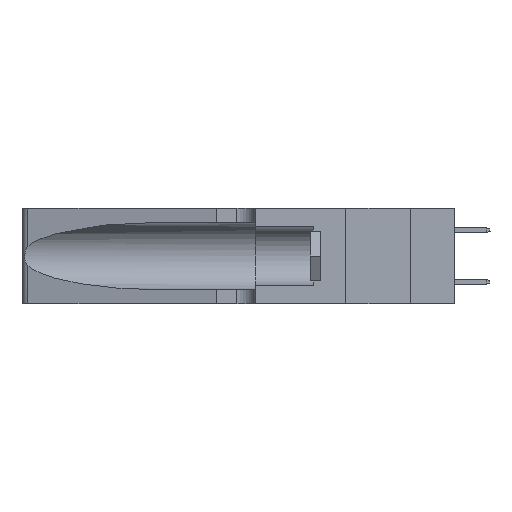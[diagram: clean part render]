
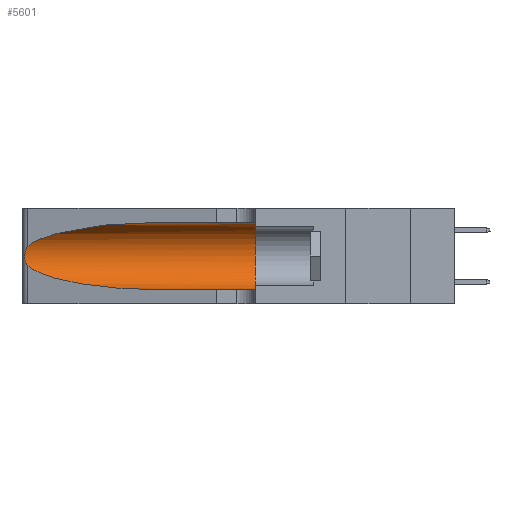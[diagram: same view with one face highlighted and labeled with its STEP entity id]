
A CAD part, left-side view. The second image highlights one B-rep face of the part: STEP entity #5601.
In plain terms, the highlighted cylindrical face has radius 3.308 mm (diameter 6.617 mm), a partial arc.
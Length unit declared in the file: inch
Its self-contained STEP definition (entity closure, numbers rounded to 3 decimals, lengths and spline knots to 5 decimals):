
#355 = DIRECTION ( 'NONE',  ( 0., 0., -1. ) ) ;
#738 = CARTESIAN_POINT ( 'NONE',  ( 0.1305, 0.72297, 0.05475 ) ) ;
#1332 = DIRECTION ( 'NONE',  ( 0., -1., 0. ) ) ;
#1374 = CARTESIAN_POINT ( 'NONE',  ( 0.25854, 1.2359, 0.20912 ) ) ;
#2296 = ORIENTED_EDGE ( 'NONE', *, *, #19547, .F. ) ;
#2709 = AXIS2_PLACEMENT_3D ( 'NONE', #27264, #29371, #355 ) ;
#2845 = B_SPLINE_CURVE_WITH_KNOTS ( 'NONE', 3,
 ( #17600, #26781, #13223, #26329, #1374, #10476, #26480, #7407, #28052, #5335, #20280, #6731, #5182, #7554 ),
 .UNSPECIFIED., .F., .F.,
 ( 4, 2, 2, 2, 2, 2, 4 ),
 ( 0., 0.00027, 0.00053, 0.00107, 0.0016, 0.00187, 0.00214 ),
 .UNSPECIFIED. ) ;
#2943 = ORIENTED_EDGE ( 'NONE', *, *, #17723, .F. ) ;
#3003 = VERTEX_POINT ( 'NONE', #13930 ) ;
#3136 = CARTESIAN_POINT ( 'NONE',  ( 0.1305, 0.72297, 0.31525 ) ) ;
#3409 = CARTESIAN_POINT ( 'NONE',  ( 0.1305, 0.72297, 0.05475 ) ) ;
#4041 = VECTOR ( 'NONE', #1332, 39.37008 ) ;
#4265 = CARTESIAN_POINT ( 'NONE',  ( 0.18966, 0.96281, 0.31525 ) ) ;
#4779 = DIRECTION ( 'NONE',  ( 0., 1., 0. ) ) ;
#5169 = VERTEX_POINT ( 'NONE', #26690 ) ;
#5182 = CARTESIAN_POINT ( 'NONE',  ( 0.25555, 1.22993, 0.14849 ) ) ;
#5335 = CARTESIAN_POINT ( 'NONE',  ( 0.25856, 1.23593, 0.16098 ) ) ;
#5574 = EDGE_CURVE ( 'NONE', #22868, #11970, #13783, .T. ) ;
#5601 = ADVANCED_FACE ( 'NONE', ( #20497 ), #17951, .F. ) ;
#5911 = CARTESIAN_POINT ( 'NONE',  ( 0.25487, 1.22718, 0.22369 ) ) ;
#6731 = CARTESIAN_POINT ( 'NONE',  ( 0.25639, 1.23186, 0.15144 ) ) ;
#7407 = CARTESIAN_POINT ( 'NONE',  ( 0.26075, 1.23896, 0.178 ) ) ;
#7554 = CARTESIAN_POINT ( 'NONE',  ( 0.25487, 1.22718, 0.14631 ) ) ;
#8176 = EDGE_CURVE ( 'NONE', #11970, #15754, #2845, .T. ) ;
#8740 = CARTESIAN_POINT ( 'NONE',  ( 0.25487, 1.22718, 0.22369 ) ) ;
#9596 = EDGE_LOOP ( 'NONE', ( #29427, #20865, #21105, #21222, #2296, #2943 ) ) ;
#10476 = CARTESIAN_POINT ( 'NONE',  ( 0.26018, 1.23835, 0.19895 ) ) ;
#10691 = CARTESIAN_POINT ( 'NONE',  ( 0.2373, 1.15595, 0.28018 ) ) ;
#11322 = LINE ( 'NONE', #15415, #26388 ) ;
#11472 = DIRECTION ( 'NONE',  ( 0., 0., 1. ) ) ;
#11597 = DIRECTION ( 'NONE',  ( 0., -1., 0. ) ) ;
#11970 = VERTEX_POINT ( 'NONE', #8740 ) ;
#13223 = CARTESIAN_POINT ( 'NONE',  ( 0.25639, 1.23184, 0.21858 ) ) ;
#13783 =( BOUNDED_CURVE ( )  B_SPLINE_CURVE ( 3, ( #24149, #4265, #10691, #5911 ),
 .UNSPECIFIED., .F., .F. ) 
 B_SPLINE_CURVE_WITH_KNOTS ( ( 4, 4 ),
 ( 1.5708, 2.84003 ),
 .UNSPECIFIED. ) 
 CURVE ( )  GEOMETRIC_REPRESENTATION_ITEM ( )  RATIONAL_B_SPLINE_CURVE ( ( 1., 0.87, 0.87, 1. ) ) 
 REPRESENTATION_ITEM ( '' )  );
#13930 = CARTESIAN_POINT ( 'NONE',  ( 0.1305, 0.35, 0.05475 ) ) ;
#15415 = CARTESIAN_POINT ( 'NONE',  ( 0.1305, 1.61858, 0.31525 ) ) ;
#15754 = VERTEX_POINT ( 'NONE', #26516 ) ;
#17111 = CARTESIAN_POINT ( 'NONE',  ( 0.25487, 1.22718, 0.14631 ) ) ;
#17600 = CARTESIAN_POINT ( 'NONE',  ( 0.25487, 1.22718, 0.22369 ) ) ;
#17723 = EDGE_CURVE ( 'NONE', #22868, #5169, #11322, .T. ) ;
#17951 = CYLINDRICAL_SURFACE ( 'NONE', #2709, 0.13025 ) ;
#18753 = CIRCLE ( 'NONE', #22146, 0.13025 ) ;
#18941 =( BOUNDED_CURVE ( )  B_SPLINE_CURVE ( 3, ( #17111, #26122, #26288, #3409 ),
 .UNSPECIFIED., .F., .T. ) 
 B_SPLINE_CURVE_WITH_KNOTS ( ( 4, 4 ),
 ( 3.44316, 4.71239 ),
 .UNSPECIFIED. ) 
 CURVE ( )  GEOMETRIC_REPRESENTATION_ITEM ( )  RATIONAL_B_SPLINE_CURVE ( ( 1., 0.87, 0.87, 1. ) ) 
 REPRESENTATION_ITEM ( '' )  );
#19547 = EDGE_CURVE ( 'NONE', #5169, #3003, #18753, .T. ) ;
#20280 = CARTESIAN_POINT ( 'NONE',  ( 0.25789, 1.23486, 0.15765 ) ) ;
#20497 = FACE_OUTER_BOUND ( 'NONE', #9596, .T. ) ;
#20865 = ORIENTED_EDGE ( 'NONE', *, *, #8176, .T. ) ;
#21105 = ORIENTED_EDGE ( 'NONE', *, *, #21432, .T. ) ;
#21222 = ORIENTED_EDGE ( 'NONE', *, *, #21434, .T. ) ;
#21432 = EDGE_CURVE ( 'NONE', #15754, #23344, #18941, .T. ) ;
#21434 = EDGE_CURVE ( 'NONE', #23344, #3003, #23885, .T. ) ;
#21782 = CARTESIAN_POINT ( 'NONE',  ( 0.1305, 1.61858, 0.05475 ) ) ;
#22146 = AXIS2_PLACEMENT_3D ( 'NONE', #25250, #4779, #11472 ) ;
#22868 = VERTEX_POINT ( 'NONE', #3136 ) ;
#23344 = VERTEX_POINT ( 'NONE', #738 ) ;
#23885 = LINE ( 'NONE', #21782, #4041 ) ;
#24149 = CARTESIAN_POINT ( 'NONE',  ( 0.1305, 0.72297, 0.31525 ) ) ;
#25250 = CARTESIAN_POINT ( 'NONE',  ( 0.1305, 0.35, 0.185 ) ) ;
#26122 = CARTESIAN_POINT ( 'NONE',  ( 0.2373, 1.15595, 0.08982 ) ) ;
#26288 = CARTESIAN_POINT ( 'NONE',  ( 0.18966, 0.96281, 0.05475 ) ) ;
#26329 = CARTESIAN_POINT ( 'NONE',  ( 0.25787, 1.23484, 0.2124 ) ) ;
#26388 = VECTOR ( 'NONE', #11597, 39.37008 ) ;
#26480 = CARTESIAN_POINT ( 'NONE',  ( 0.26075, 1.23896, 0.19203 ) ) ;
#26516 = CARTESIAN_POINT ( 'NONE',  ( 0.25487, 1.22718, 0.14631 ) ) ;
#26690 = CARTESIAN_POINT ( 'NONE',  ( 0.1305, 0.35, 0.31525 ) ) ;
#26781 = CARTESIAN_POINT ( 'NONE',  ( 0.25555, 1.22994, 0.2215 ) ) ;
#27264 = CARTESIAN_POINT ( 'NONE',  ( 0.1305, 1.61858, 0.185 ) ) ;
#28052 = CARTESIAN_POINT ( 'NONE',  ( 0.26017, 1.23833, 0.17102 ) ) ;
#29371 = DIRECTION ( 'NONE',  ( 0., -1., 0. ) ) ;
#29427 = ORIENTED_EDGE ( 'NONE', *, *, #5574, .T. ) ;
